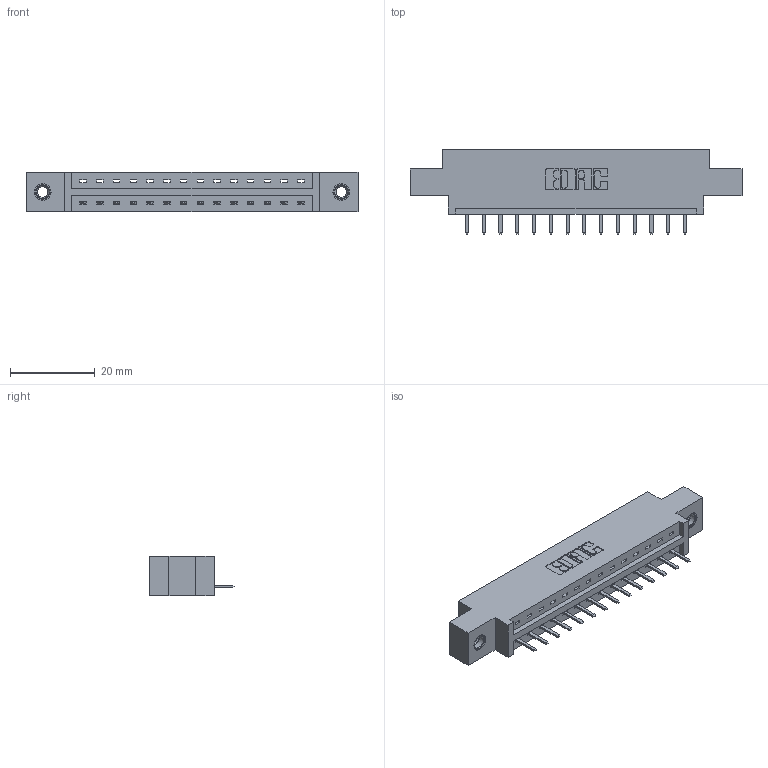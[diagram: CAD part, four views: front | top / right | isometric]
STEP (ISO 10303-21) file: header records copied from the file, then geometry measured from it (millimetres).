
FILE_DESCRIPTION (( 'STEP AP203' ), '1' );
FILE_NAME ('337-014-520-607.STEP', '2018-08-04T13:57:22', ( '' ), ( '' ), 'SwSTEP 2.0', 'SolidWorks 2016', '' );
FILE_SCHEMA (( 'CONFIG_CONTROL_DESIGN' ));
Length unit declared in the file: inch
Products named in the file (4): 337 Part_0.170 Offset - 0.156 Dia-TI; 345-292-001_345-293-120; 345-250-001_345-250-005-103; 337-014-520-607
Assembly tree (17 placements, depth 2):
  337-014-520-607
    337 Part_0.170 Offset - 0.156 Dia-TI
    345-292-001_345-293-120  x14
    345-250-001_345-250-005-103  x2
Bounding box: 78.49 x 20.02 x 9.4 mm (x, y, z)
Volume: 7635.6 mm3; surface area: 7727.4 mm2
Topology: 17 solids, 17 shells, 1102 faces, 3203 edges, 2090 vertices
Faces by surface type: plane 778, cylinder 308, cone 12, torus 4
Entity records: 15460 total; most frequent: CARTESIAN_POINT 2683, ORIENTED_EDGE 2614, DIRECTION 2337, EDGE_CURVE 1307, LINE 1155, VECTOR 1155, VERTEX_POINT 864, AXIS2_PLACEMENT_3D 591
